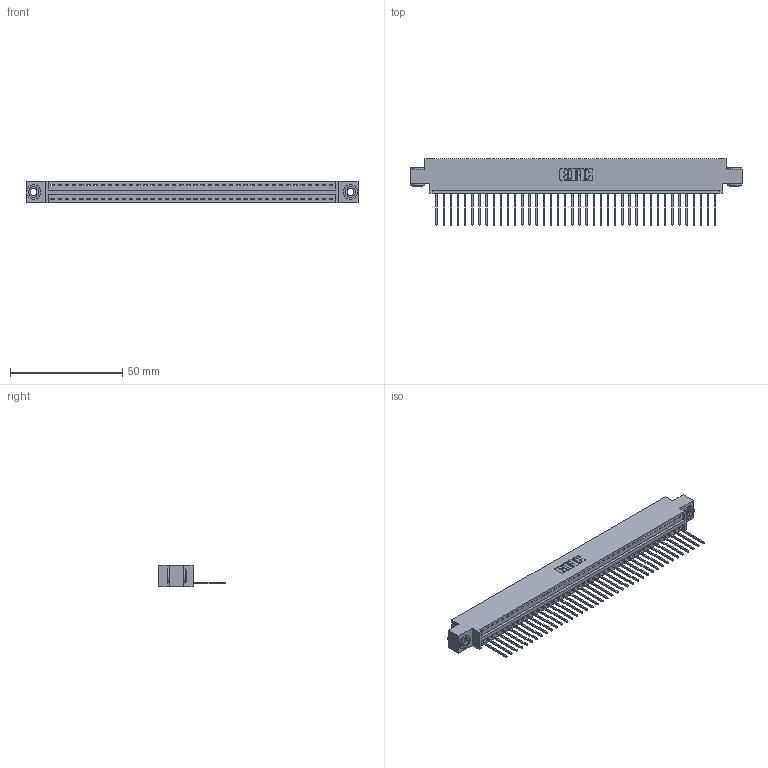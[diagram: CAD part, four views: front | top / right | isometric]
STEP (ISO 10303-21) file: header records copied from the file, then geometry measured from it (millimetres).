
FILE_DESCRIPTION (( 'STEP AP203' ), '1' );
FILE_NAME ('346-040-540-603.STEP', '2022-05-07T09:48:24', ( '' ), ( '' ), 'SwSTEP 2.0', 'SolidWorks 2020', '' );
FILE_SCHEMA (( 'CONFIG_CONTROL_DESIGN' ));
Length unit declared in the file: inch
Products named in the file (4): 345-250-002_345-250-002-102; 346-040-540-603; 346 Part_0.170 Offset - 0.156 Dia-TH; 345-292-001_345-293-140
Assembly tree (43 placements, depth 2):
  346-040-540-603
    346 Part_0.170 Offset - 0.156 Dia-TH
    345-292-001_345-293-140  x40
    345-250-002_345-250-002-102  x2
Bounding box: 147.57 x 29.46 x 9.4 mm (x, y, z)
Volume: 14013.2 mm3; surface area: 18300.3 mm2
Topology: 43 solids, 43 shells, 2498 faces, 7493 edges, 4938 vertices
Faces by surface type: plane 1704, cylinder 786, cone 8
Entity records: 26310 total; most frequent: CARTESIAN_POINT 4493, ORIENTED_EDGE 4458, DIRECTION 3995, EDGE_CURVE 2229, VECTOR 1913, LINE 1913, VERTEX_POINT 1482, AXIS2_PLACEMENT_3D 1041
